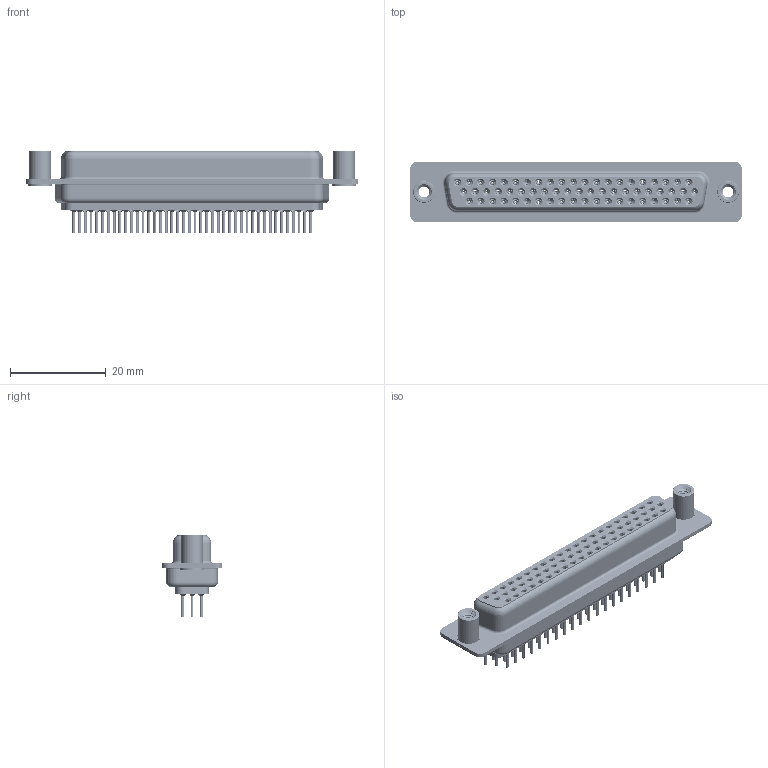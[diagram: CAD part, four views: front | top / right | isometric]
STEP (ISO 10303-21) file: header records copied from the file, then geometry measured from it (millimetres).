
FILE_DESCRIPTION (( 'STEP AP203' ), '1' );
FILE_NAME ('638-062-230-248.STEP', '2020-07-19T00:50:07', ( '' ), ( '' ), 'SwSTEP 2.0', 'SolidWorks 2020', '' );
FILE_SCHEMA (( 'CONFIG_CONTROL_DESIGN' ));
Length unit declared in the file: millimetre
Products named in the file (8): 638 Shell Rear_62 Contacts; 638 Contact Row 2_30; 638-062-230-248; 638 Housing_62 Contacts; 638 Contact Row 3_30; 638 Shell Front_62 Contacts; 638 4-40 Threaded Standoff; 638 Contact Row 1_30
Assembly tree (67 placements, depth 2):
  638-062-230-248
    638 Housing_62 Contacts
    638 Shell Front_62 Contacts
    638 Shell Rear_62 Contacts
    638 Contact Row 1_30  x21
    638 Contact Row 2_30  x21
    638 Contact Row 3_30  x20
    638 4-40 Threaded Standoff  x2
Bounding box: 69.32 x 12.6 x 17.3 mm (x, y, z)
Volume: 4659.4 mm3; surface area: 17655.7 mm2
Topology: 67 solids, 67 shells, 8187 faces, 20865 edges, 12949 vertices
Faces by surface type: cylinder 2211, plane 1991, torus 1669, bspline 1246, cone 1070
Entity records: 47758 total; most frequent: CARTESIAN_POINT 12293, DIRECTION 7404, ORIENTED_EDGE 6518, EDGE_CURVE 3259, AXIS2_PLACEMENT_3D 3131, VERTEX_POINT 2064, EDGE_LOOP 1739, CIRCLE 1719
